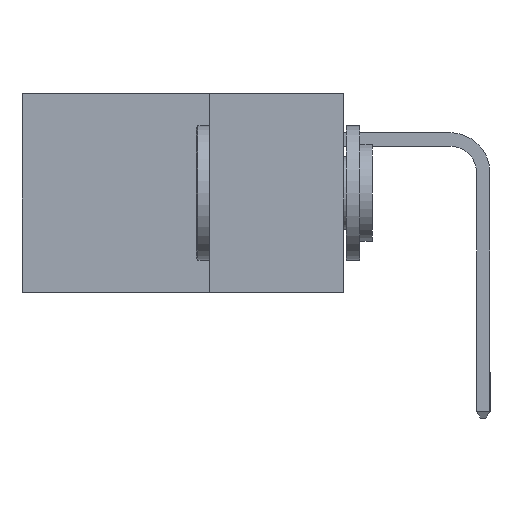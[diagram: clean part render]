
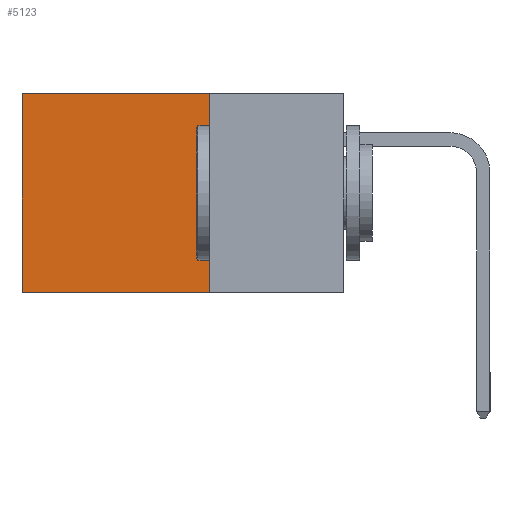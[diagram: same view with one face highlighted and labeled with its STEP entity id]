
A CAD part, left-side view. The second image highlights one B-rep face of the part: STEP entity #5123.
In plain terms, the highlighted planar face has unit normal (-1, 0, 0).
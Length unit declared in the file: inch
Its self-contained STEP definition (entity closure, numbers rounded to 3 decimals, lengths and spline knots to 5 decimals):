
#367 = LINE ( 'NONE', #4212, #7914 ) ;
#1434 = VERTEX_POINT ( 'NONE', #4006 ) ;
#1645 = DIRECTION ( 'NONE',  ( 0., 1., 0. ) ) ;
#1754 = VECTOR ( 'NONE', #1645, 39.37008 ) ;
#1886 = VECTOR ( 'NONE', #5370, 39.37008 ) ;
#2649 = CARTESIAN_POINT ( 'NONE',  ( 0.2615, 0.25, -0.37 ) ) ;
#2746 = LINE ( 'NONE', #10542, #11153 ) ;
#2829 = EDGE_CURVE ( 'NONE', #1434, #8437, #10271, .T. ) ;
#2945 = ORIENTED_EDGE ( 'NONE', *, *, #2829, .F. ) ;
#2984 = DIRECTION ( 'NONE',  ( 1., 0., 0. ) ) ;
#3658 = VERTEX_POINT ( 'NONE', #7211 ) ;
#4006 = CARTESIAN_POINT ( 'NONE',  ( 0.2615, 0.25, -0.37 ) ) ;
#4212 = CARTESIAN_POINT ( 'NONE',  ( 0.2615, 0.25, -0.37 ) ) ;
#4551 = CARTESIAN_POINT ( 'NONE',  ( 0.2615, 0.25, 0. ) ) ;
#4977 = EDGE_CURVE ( 'NONE', #6087, #8437, #2746, .T. ) ;
#5028 = CARTESIAN_POINT ( 'NONE',  ( 0.2615, 0.6, 0. ) ) ;
#5123 = ADVANCED_FACE ( 'NONE', ( #7767 ), #9838, .F. ) ;
#5154 = ORIENTED_EDGE ( 'NONE', *, *, #6225, .F. ) ;
#5370 = DIRECTION ( 'NONE',  ( 0., 1., 0. ) ) ;
#6087 = VERTEX_POINT ( 'NONE', #5028 ) ;
#6225 = EDGE_CURVE ( 'NONE', #3658, #1434, #367, .T. ) ;
#6646 = DIRECTION ( 'NONE',  ( 0., 0., -1. ) ) ;
#7211 = CARTESIAN_POINT ( 'NONE',  ( 0.2615, 0.25, 0. ) ) ;
#7767 = FACE_OUTER_BOUND ( 'NONE', #8396, .T. ) ;
#7914 = VECTOR ( 'NONE', #11884, 39.37008 ) ;
#8248 = ORIENTED_EDGE ( 'NONE', *, *, #9571, .T. ) ;
#8396 = EDGE_LOOP ( 'NONE', ( #12380, #2945, #5154, #8248 ) ) ;
#8437 = VERTEX_POINT ( 'NONE', #9567 ) ;
#8538 = AXIS2_PLACEMENT_3D ( 'NONE', #8887, #2984, #10674 ) ;
#8887 = CARTESIAN_POINT ( 'NONE',  ( 0.2615, 0.25, -0.37 ) ) ;
#9567 = CARTESIAN_POINT ( 'NONE',  ( 0.2615, 0.6, -0.37 ) ) ;
#9571 = EDGE_CURVE ( 'NONE', #3658, #6087, #10278, .T. ) ;
#9838 = PLANE ( 'NONE',  #8538 ) ;
#10271 = LINE ( 'NONE', #2649, #1886 ) ;
#10278 = LINE ( 'NONE', #4551, #1754 ) ;
#10542 = CARTESIAN_POINT ( 'NONE',  ( 0.2615, 0.6, -0.37 ) ) ;
#10674 = DIRECTION ( 'NONE',  ( 0., 0., -1. ) ) ;
#11153 = VECTOR ( 'NONE', #6646, 39.37008 ) ;
#11884 = DIRECTION ( 'NONE',  ( 0., 0., -1. ) ) ;
#12380 = ORIENTED_EDGE ( 'NONE', *, *, #4977, .T. ) ;
